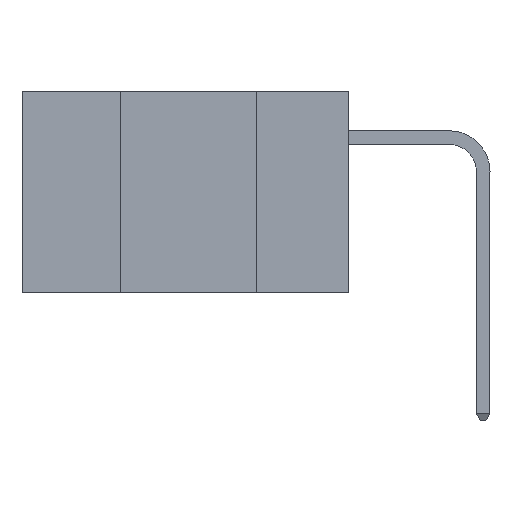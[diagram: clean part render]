
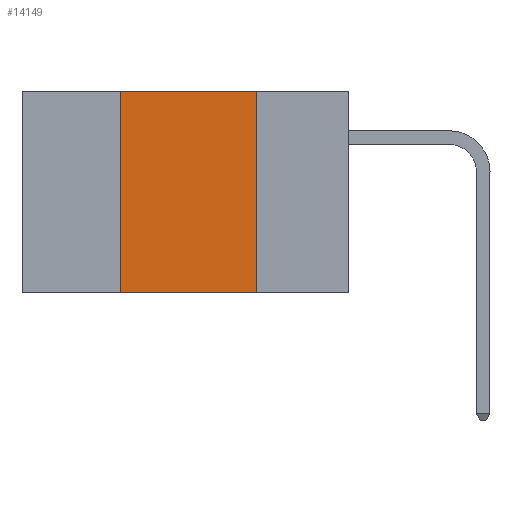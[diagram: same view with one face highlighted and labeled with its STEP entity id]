
A CAD part, left-side view. The second image highlights one B-rep face of the part: STEP entity #14149.
In plain terms, the highlighted planar face has unit normal (-1, 0, 0).
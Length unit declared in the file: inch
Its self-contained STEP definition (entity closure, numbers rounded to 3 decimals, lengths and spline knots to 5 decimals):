
#624 = AXIS2_PLACEMENT_3D ( 'NONE', #1603, #33636, #18883 ) ;
#1603 = CARTESIAN_POINT ( 'NONE',  ( 0., 0.6, 0. ) ) ;
#3959 = CARTESIAN_POINT ( 'NONE',  ( 0., 0.17, 0. ) ) ;
#3970 = ORIENTED_EDGE ( 'NONE', *, *, #24012, .T. ) ;
#4671 = EDGE_CURVE ( 'NONE', #32326, #34633, #16542, .T. ) ;
#6384 = CARTESIAN_POINT ( 'NONE',  ( 0., 0.42, 0. ) ) ;
#7124 = EDGE_LOOP ( 'NONE', ( #9434, #17245, #23277, #3970 ) ) ;
#7181 = PLANE ( 'NONE',  #624 ) ;
#8237 = EDGE_CURVE ( 'NONE', #34633, #10150, #20144, .T. ) ;
#9434 = ORIENTED_EDGE ( 'NONE', *, *, #21198, .F. ) ;
#10150 = VERTEX_POINT ( 'NONE', #3959 ) ;
#11330 = FACE_OUTER_BOUND ( 'NONE', #7124, .T. ) ;
#12776 = CARTESIAN_POINT ( 'NONE',  ( 0., 0.6, -0.37 ) ) ;
#13358 = VERTEX_POINT ( 'NONE', #30063 ) ;
#14149 = ADVANCED_FACE ( 'NONE', ( #11330 ), #7181, .F. ) ;
#16542 = LINE ( 'NONE', #6384, #28282 ) ;
#16736 = CARTESIAN_POINT ( 'NONE',  ( 0., 0.17, 0. ) ) ;
#17123 = CARTESIAN_POINT ( 'NONE',  ( 0., 0.42, 0. ) ) ;
#17245 = ORIENTED_EDGE ( 'NONE', *, *, #8237, .F. ) ;
#18191 = VECTOR ( 'NONE', #24635, 39.37008 ) ;
#18883 = DIRECTION ( 'NONE',  ( 0., 0., -1. ) ) ;
#19262 = CARTESIAN_POINT ( 'NONE',  ( 0., 0.6, 0. ) ) ;
#20144 = LINE ( 'NONE', #19262, #32764 ) ;
#20878 = DIRECTION ( 'NONE',  ( 0., 0., 1. ) ) ;
#21198 = EDGE_CURVE ( 'NONE', #10150, #13358, #26179, .T. ) ;
#23277 = ORIENTED_EDGE ( 'NONE', *, *, #4671, .F. ) ;
#24012 = EDGE_CURVE ( 'NONE', #32326, #13358, #24083, .T. ) ;
#24083 = LINE ( 'NONE', #12776, #18191 ) ;
#24635 = DIRECTION ( 'NONE',  ( 0., -1., 0. ) ) ;
#26179 = LINE ( 'NONE', #16736, #34265 ) ;
#27602 = DIRECTION ( 'NONE',  ( 0., -1., 0. ) ) ;
#28282 = VECTOR ( 'NONE', #20878, 39.37008 ) ;
#30063 = CARTESIAN_POINT ( 'NONE',  ( 0., 0.17, -0.37 ) ) ;
#31534 = CARTESIAN_POINT ( 'NONE',  ( 0., 0.42, -0.37 ) ) ;
#32326 = VERTEX_POINT ( 'NONE', #31534 ) ;
#32764 = VECTOR ( 'NONE', #27602, 39.37008 ) ;
#33636 = DIRECTION ( 'NONE',  ( 1., 0., 0. ) ) ;
#34265 = VECTOR ( 'NONE', #36927, 39.37008 ) ;
#34633 = VERTEX_POINT ( 'NONE', #17123 ) ;
#36927 = DIRECTION ( 'NONE',  ( 0., 0., -1. ) ) ;
